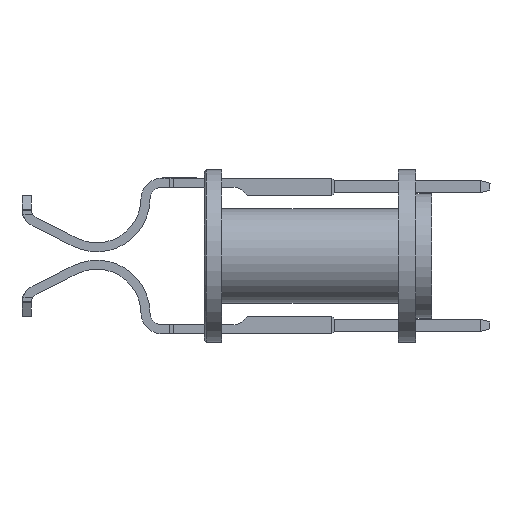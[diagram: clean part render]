
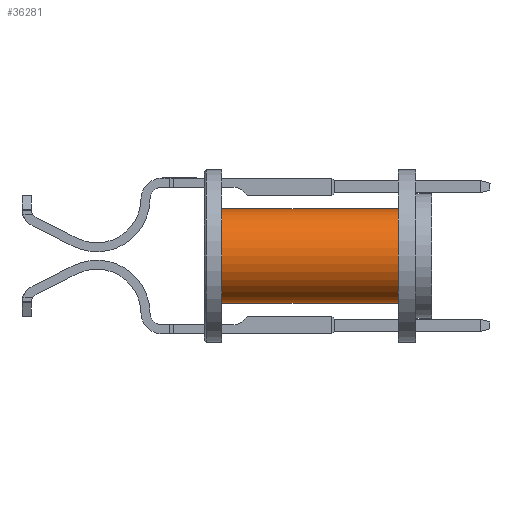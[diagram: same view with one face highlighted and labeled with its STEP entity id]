
A CAD part, left-side view. The second image highlights one B-rep face of the part: STEP entity #36281.
In plain terms, the highlighted cylindrical face has radius 1.727 mm (diameter 3.454 mm), a partial arc.
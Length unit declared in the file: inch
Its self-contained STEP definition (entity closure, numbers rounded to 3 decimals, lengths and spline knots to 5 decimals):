
#3599 = VERTEX_POINT ( 'NONE', #7019 ) ;
#4825 = AXIS2_PLACEMENT_3D ( 'NONE', #16463, #32308, #25221 ) ;
#4875 = EDGE_CURVE ( 'NONE', #11692, #14810, #7281, .T. ) ;
#5640 = EDGE_LOOP ( 'NONE', ( #23628, #11946, #49023, #11771 ) ) ;
#6739 = LINE ( 'NONE', #7501, #26036 ) ;
#7006 = EDGE_CURVE ( 'NONE', #3599, #43514, #7316, .T. ) ;
#7019 = CARTESIAN_POINT ( 'NONE',  ( 0., 0.025, 0.068 ) ) ;
#7281 = CIRCLE ( 'NONE', #4825, 0.068 ) ;
#7316 = CIRCLE ( 'NONE', #27258, 0.068 ) ;
#7501 = CARTESIAN_POINT ( 'NONE',  ( 0., 0.328, 0.068 ) ) ;
#11692 = VERTEX_POINT ( 'NONE', #23702 ) ;
#11771 = ORIENTED_EDGE ( 'NONE', *, *, #30392, .F. ) ;
#11946 = ORIENTED_EDGE ( 'NONE', *, *, #20336, .T. ) ;
#14810 = VERTEX_POINT ( 'NONE', #43640 ) ;
#16463 = CARTESIAN_POINT ( 'NONE',  ( 0., 0.28, 0. ) ) ;
#16963 = CARTESIAN_POINT ( 'NONE',  ( 0., 0.328, 0. ) ) ;
#18851 = DIRECTION ( 'NONE',  ( 0., 0., 1. ) ) ;
#20336 = EDGE_CURVE ( 'NONE', #11692, #3599, #6739, .T. ) ;
#21642 = FACE_OUTER_BOUND ( 'NONE', #5640, .T. ) ;
#23628 = ORIENTED_EDGE ( 'NONE', *, *, #4875, .F. ) ;
#23702 = CARTESIAN_POINT ( 'NONE',  ( 0., 0.28, 0.068 ) ) ;
#24516 = CYLINDRICAL_SURFACE ( 'NONE', #35650, 0.068 ) ;
#25221 = DIRECTION ( 'NONE',  ( 0., 0., 1. ) ) ;
#26036 = VECTOR ( 'NONE', #30904, 39.37008 ) ;
#26609 = VECTOR ( 'NONE', #40227, 39.37008 ) ;
#27258 = AXIS2_PLACEMENT_3D ( 'NONE', #42998, #30299, #18851 ) ;
#29268 = CARTESIAN_POINT ( 'NONE',  ( 0., 0.025, -0.068 ) ) ;
#30299 = DIRECTION ( 'NONE',  ( 0., 1., 0. ) ) ;
#30392 = EDGE_CURVE ( 'NONE', #14810, #43514, #44148, .T. ) ;
#30904 = DIRECTION ( 'NONE',  ( 0., -1., 0. ) ) ;
#32308 = DIRECTION ( 'NONE',  ( 0., 1., 0. ) ) ;
#35650 = AXIS2_PLACEMENT_3D ( 'NONE', #16963, #49421, #45276 ) ;
#36281 = ADVANCED_FACE ( 'NONE', ( #21642 ), #24516, .T. ) ;
#40227 = DIRECTION ( 'NONE',  ( 0., -1., 0. ) ) ;
#40752 = CARTESIAN_POINT ( 'NONE',  ( 0., 0.328, -0.068 ) ) ;
#42998 = CARTESIAN_POINT ( 'NONE',  ( 0., 0.025, 0. ) ) ;
#43514 = VERTEX_POINT ( 'NONE', #29268 ) ;
#43640 = CARTESIAN_POINT ( 'NONE',  ( 0., 0.28, -0.068 ) ) ;
#44148 = LINE ( 'NONE', #40752, #26609 ) ;
#45276 = DIRECTION ( 'NONE',  ( 0., 0., -1. ) ) ;
#49023 = ORIENTED_EDGE ( 'NONE', *, *, #7006, .T. ) ;
#49421 = DIRECTION ( 'NONE',  ( 0., -1., 0. ) ) ;
